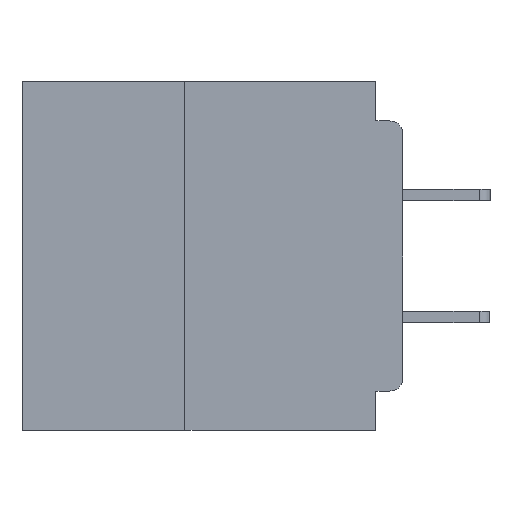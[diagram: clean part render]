
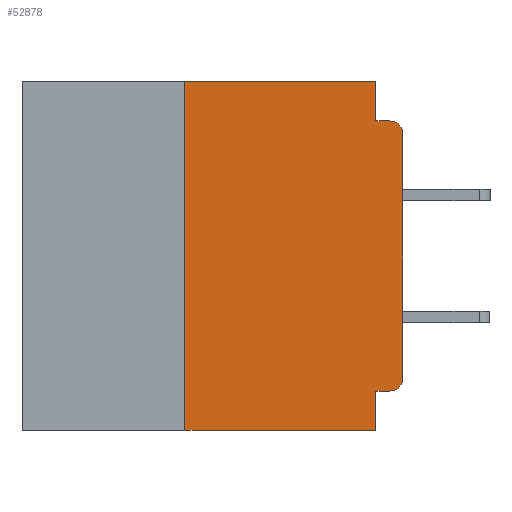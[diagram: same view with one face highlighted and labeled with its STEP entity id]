
A CAD part, left-side view. The second image highlights one B-rep face of the part: STEP entity #52878.
In plain terms, the highlighted planar face has unit normal (-1, 0, 0).
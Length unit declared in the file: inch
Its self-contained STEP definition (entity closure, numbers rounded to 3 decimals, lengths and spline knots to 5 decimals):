
#1915 = DIRECTION ( 'NONE',  ( 0., 1., 0. ) ) ;
#2029 = CARTESIAN_POINT ( 'NONE',  ( 0., 0., -0.06 ) ) ;
#2294 = DIRECTION ( 'NONE',  ( 0., 0., 1. ) ) ;
#2888 = DIRECTION ( 'NONE',  ( 0., 0., -1. ) ) ;
#3358 = VECTOR ( 'NONE', #36472, 39.37008 ) ;
#4114 = VECTOR ( 'NONE', #56252, 39.37008 ) ;
#4355 = ORIENTED_EDGE ( 'NONE', *, *, #42667, .F. ) ;
#5793 = ORIENTED_EDGE ( 'NONE', *, *, #25449, .F. ) ;
#6490 = VERTEX_POINT ( 'NONE', #38612 ) ;
#6760 = CARTESIAN_POINT ( 'NONE',  ( 0., 0., -0.34 ) ) ;
#7682 = EDGE_CURVE ( 'NONE', #11304, #15137, #44916, .T. ) ;
#8917 = DIRECTION ( 'NONE',  ( 1., 0., 0. ) ) ;
#9316 = VERTEX_POINT ( 'NONE', #53293 ) ;
#9620 = VECTOR ( 'NONE', #54828, 39.37008 ) ;
#9776 = CARTESIAN_POINT ( 'NONE',  ( 0., 0.031, -0.4 ) ) ;
#9890 = CARTESIAN_POINT ( 'NONE',  ( 0., 0.437, 0. ) ) ;
#10741 = CARTESIAN_POINT ( 'NONE',  ( 0., 0.031, -0.4 ) ) ;
#10791 = CARTESIAN_POINT ( 'NONE',  ( 0., 0.015, -0.06 ) ) ;
#11304 = VERTEX_POINT ( 'NONE', #17482 ) ;
#13179 = CARTESIAN_POINT ( 'NONE',  ( 0., 0.437, 0. ) ) ;
#13194 = AXIS2_PLACEMENT_3D ( 'NONE', #55932, #29480, #2888 ) ;
#13274 = ORIENTED_EDGE ( 'NONE', *, *, #38630, .F. ) ;
#14932 = EDGE_LOOP ( 'NONE', ( #49445, #48560, #13274, #36957, #5793, #53804, #32591, #36681, #4355, #20642 ) ) ;
#14936 = CARTESIAN_POINT ( 'NONE',  ( 0., 0.437, -0.4 ) ) ;
#15137 = VERTEX_POINT ( 'NONE', #9776 ) ;
#15185 = LINE ( 'NONE', #9890, #3358 ) ;
#15229 = DIRECTION ( 'NONE',  ( 0., 0., -1. ) ) ;
#15955 = LINE ( 'NONE', #34087, #4114 ) ;
#15956 = EDGE_CURVE ( 'NONE', #9316, #35025, #50418, .T. ) ;
#16270 = LINE ( 'NONE', #50704, #47661 ) ;
#16716 = EDGE_CURVE ( 'NONE', #35025, #21300, #44086, .T. ) ;
#17482 = CARTESIAN_POINT ( 'NONE',  ( 0., 0.031, -0.355 ) ) ;
#20642 = ORIENTED_EDGE ( 'NONE', *, *, #15956, .T. ) ;
#21300 = VERTEX_POINT ( 'NONE', #2029 ) ;
#21617 = FACE_OUTER_BOUND ( 'NONE', #14932, .T. ) ;
#21946 = LINE ( 'NONE', #42070, #44068 ) ;
#23066 = AXIS2_PLACEMENT_3D ( 'NONE', #10791, #41770, #15229 ) ;
#24086 = CARTESIAN_POINT ( 'NONE',  ( 0., 0., -0.355 ) ) ;
#24321 = VERTEX_POINT ( 'NONE', #34297 ) ;
#25449 = EDGE_CURVE ( 'NONE', #56369, #24321, #15185, .T. ) ;
#25530 = EDGE_CURVE ( 'NONE', #6490, #15137, #34607, .T. ) ;
#26535 = PLANE ( 'NONE',  #51192 ) ;
#27091 = DIRECTION ( 'NONE',  ( 0., 0., 1. ) ) ;
#27093 = LINE ( 'NONE', #24086, #49229 ) ;
#27380 = CARTESIAN_POINT ( 'NONE',  ( 0., 0.015, -0.045 ) ) ;
#29480 = DIRECTION ( 'NONE',  ( -1., 0., 0. ) ) ;
#31293 = VERTEX_POINT ( 'NONE', #40917 ) ;
#31474 = EDGE_CURVE ( 'NONE', #6490, #56369, #21946, .T. ) ;
#32562 = DIRECTION ( 'NONE',  ( 0., -1., 0. ) ) ;
#32591 = ORIENTED_EDGE ( 'NONE', *, *, #25530, .T. ) ;
#33227 = VECTOR ( 'NONE', #32562, 39.37008 ) ;
#33798 = EDGE_CURVE ( 'NONE', #21300, #52379, #54027, .T. ) ;
#34087 = CARTESIAN_POINT ( 'NONE',  ( 0., 0.031, 0. ) ) ;
#34297 = CARTESIAN_POINT ( 'NONE',  ( 0., 0.031, 0. ) ) ;
#34607 = LINE ( 'NONE', #14936, #33227 ) ;
#35025 = VERTEX_POINT ( 'NONE', #6760 ) ;
#35857 = CARTESIAN_POINT ( 'NONE',  ( 0., 0., 0. ) ) ;
#36472 = DIRECTION ( 'NONE',  ( 0., -1., 0. ) ) ;
#36681 = ORIENTED_EDGE ( 'NONE', *, *, #7682, .F. ) ;
#36957 = ORIENTED_EDGE ( 'NONE', *, *, #43338, .F. ) ;
#38612 = CARTESIAN_POINT ( 'NONE',  ( 0., 0.25, -0.4 ) ) ;
#38630 = EDGE_CURVE ( 'NONE', #31293, #52379, #16270, .T. ) ;
#39933 = DIRECTION ( 'NONE',  ( 0., 0., -1. ) ) ;
#40917 = CARTESIAN_POINT ( 'NONE',  ( 0., 0.031, -0.045 ) ) ;
#41770 = DIRECTION ( 'NONE',  ( -1., 0., 0. ) ) ;
#42070 = CARTESIAN_POINT ( 'NONE',  ( 0., 0.25, -0.4 ) ) ;
#42667 = EDGE_CURVE ( 'NONE', #9316, #11304, #27093, .T. ) ;
#42725 = VECTOR ( 'NONE', #27091, 39.37008 ) ;
#43338 = EDGE_CURVE ( 'NONE', #24321, #31293, #15955, .T. ) ;
#44068 = VECTOR ( 'NONE', #2294, 39.37008 ) ;
#44086 = LINE ( 'NONE', #35857, #42725 ) ;
#44916 = LINE ( 'NONE', #10741, #9620 ) ;
#45873 = CARTESIAN_POINT ( 'NONE',  ( 0., 0.25, 0. ) ) ;
#46432 = DIRECTION ( 'NONE',  ( 0., -1., 0. ) ) ;
#47661 = VECTOR ( 'NONE', #46432, 39.37008 ) ;
#48560 = ORIENTED_EDGE ( 'NONE', *, *, #33798, .T. ) ;
#49229 = VECTOR ( 'NONE', #1915, 39.37008 ) ;
#49445 = ORIENTED_EDGE ( 'NONE', *, *, #16716, .T. ) ;
#50418 = CIRCLE ( 'NONE', #13194, 0.015 ) ;
#50704 = CARTESIAN_POINT ( 'NONE',  ( 0., 0., -0.045 ) ) ;
#51192 = AXIS2_PLACEMENT_3D ( 'NONE', #13179, #8917, #39933 ) ;
#52379 = VERTEX_POINT ( 'NONE', #27380 ) ;
#52878 = ADVANCED_FACE ( 'NONE', ( #21617 ), #26535, .F. ) ;
#53293 = CARTESIAN_POINT ( 'NONE',  ( 0., 0.015, -0.355 ) ) ;
#53804 = ORIENTED_EDGE ( 'NONE', *, *, #31474, .F. ) ;
#54027 = CIRCLE ( 'NONE', #23066, 0.015 ) ;
#54828 = DIRECTION ( 'NONE',  ( 0., 0., -1. ) ) ;
#55932 = CARTESIAN_POINT ( 'NONE',  ( 0., 0.015, -0.34 ) ) ;
#56252 = DIRECTION ( 'NONE',  ( 0., 0., -1. ) ) ;
#56369 = VERTEX_POINT ( 'NONE', #45873 ) ;
